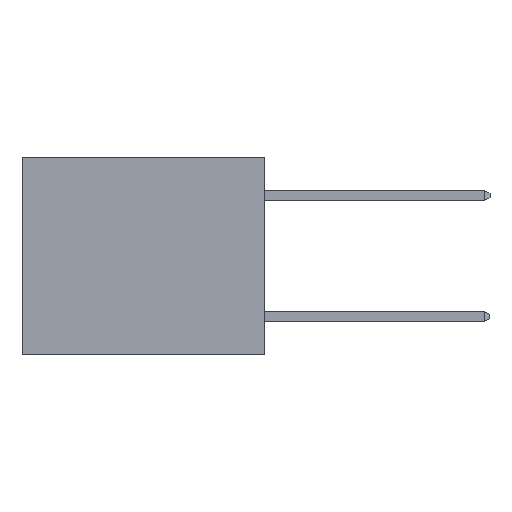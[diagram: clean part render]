
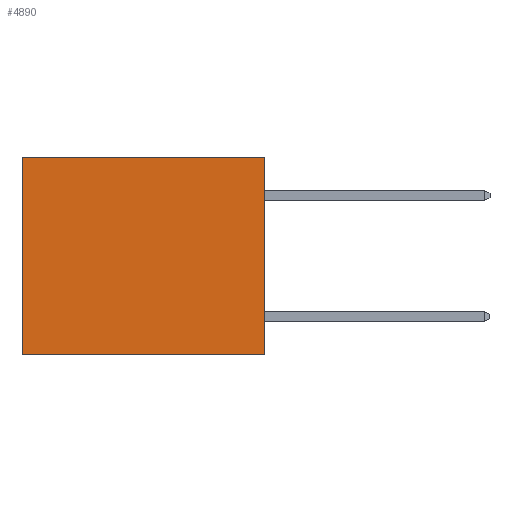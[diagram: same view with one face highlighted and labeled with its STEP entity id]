
A CAD part, left-side view. The second image highlights one B-rep face of the part: STEP entity #4890.
In plain terms, the highlighted planar face has unit normal (-1, 0, 0).
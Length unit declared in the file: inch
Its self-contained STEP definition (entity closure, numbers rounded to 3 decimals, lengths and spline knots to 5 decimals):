
#222 = DIRECTION ( 'NONE',  ( 1., 0., 0. ) ) ;
#269 = DIRECTION ( 'NONE',  ( 0., 0., -1. ) ) ;
#499 = CARTESIAN_POINT ( 'NONE',  ( 0.3165, 0.6, -0.49 ) ) ;
#874 = VECTOR ( 'NONE', #2455, 39.37008 ) ;
#1008 = VECTOR ( 'NONE', #269, 39.37008 ) ;
#1089 = VERTEX_POINT ( 'NONE', #499 ) ;
#1151 = VERTEX_POINT ( 'NONE', #3444 ) ;
#1402 = ORIENTED_EDGE ( 'NONE', *, *, #2137, .T. ) ;
#1460 = CARTESIAN_POINT ( 'NONE',  ( 0.3165, 0.6, 0. ) ) ;
#1643 = CARTESIAN_POINT ( 'NONE',  ( 0.3165, 0., 0. ) ) ;
#1663 = LINE ( 'NONE', #1643, #874 ) ;
#1940 = CARTESIAN_POINT ( 'NONE',  ( 0.3165, 0., 0. ) ) ;
#2137 = EDGE_CURVE ( 'NONE', #2520, #5361, #1663, .T. ) ;
#2395 = EDGE_CURVE ( 'NONE', #1151, #1089, #7191, .T. ) ;
#2442 = LINE ( 'NONE', #7462, #8286 ) ;
#2455 = DIRECTION ( 'NONE',  ( 0., 1., 0. ) ) ;
#2517 = ORIENTED_EDGE ( 'NONE', *, *, #6293, .F. ) ;
#2520 = VERTEX_POINT ( 'NONE', #1940 ) ;
#2822 = LINE ( 'NONE', #8806, #1008 ) ;
#3153 = CARTESIAN_POINT ( 'NONE',  ( 0.3165, 0., -0.49 ) ) ;
#3444 = CARTESIAN_POINT ( 'NONE',  ( 0.3165, 0., -0.49 ) ) ;
#4560 = DIRECTION ( 'NONE',  ( 0., 0., -1. ) ) ;
#4721 = EDGE_LOOP ( 'NONE', ( #5250, #7562, #2517, #1402 ) ) ;
#4890 = ADVANCED_FACE ( 'NONE', ( #7320 ), #7472, .F. ) ;
#5250 = ORIENTED_EDGE ( 'NONE', *, *, #9177, .T. ) ;
#5361 = VERTEX_POINT ( 'NONE', #1460 ) ;
#5437 = AXIS2_PLACEMENT_3D ( 'NONE', #3153, #222, #4560 ) ;
#5736 = DIRECTION ( 'NONE',  ( 0., 1., 0. ) ) ;
#6293 = EDGE_CURVE ( 'NONE', #2520, #1151, #2442, .T. ) ;
#6634 = DIRECTION ( 'NONE',  ( 0., 0., -1. ) ) ;
#7143 = CARTESIAN_POINT ( 'NONE',  ( 0.3165, 0., -0.49 ) ) ;
#7191 = LINE ( 'NONE', #7143, #8191 ) ;
#7320 = FACE_OUTER_BOUND ( 'NONE', #4721, .T. ) ;
#7462 = CARTESIAN_POINT ( 'NONE',  ( 0.3165, 0., -0.49 ) ) ;
#7472 = PLANE ( 'NONE',  #5437 ) ;
#7562 = ORIENTED_EDGE ( 'NONE', *, *, #2395, .F. ) ;
#8191 = VECTOR ( 'NONE', #5736, 39.37008 ) ;
#8286 = VECTOR ( 'NONE', #6634, 39.37008 ) ;
#8806 = CARTESIAN_POINT ( 'NONE',  ( 0.3165, 0.6, -0.49 ) ) ;
#9177 = EDGE_CURVE ( 'NONE', #5361, #1089, #2822, .T. ) ;
